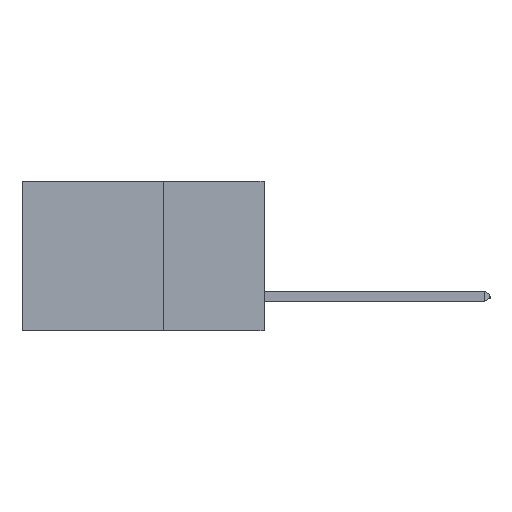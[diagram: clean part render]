
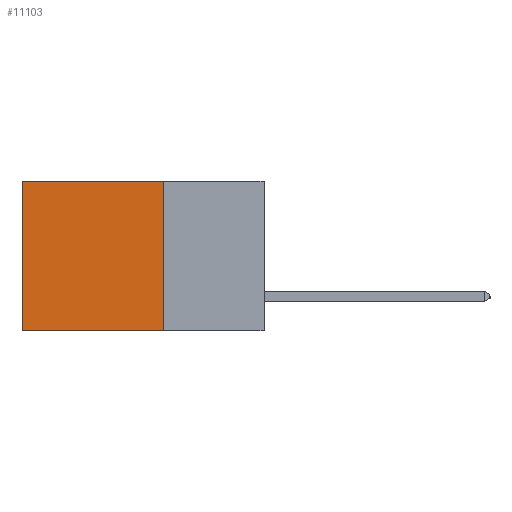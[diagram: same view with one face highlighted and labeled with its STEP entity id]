
A CAD part, left-side view. The second image highlights one B-rep face of the part: STEP entity #11103.
In plain terms, the highlighted planar face has unit normal (-1, 0, 0).
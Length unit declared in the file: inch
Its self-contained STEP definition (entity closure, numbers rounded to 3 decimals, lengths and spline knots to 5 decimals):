
#377 = DIRECTION ( 'NONE',  ( 1., 0., 0. ) ) ;
#1477 = VECTOR ( 'NONE', #22156, 39.37008 ) ;
#1693 = EDGE_CURVE ( 'NONE', #18777, #16874, #9585, .T. ) ;
#2269 = AXIS2_PLACEMENT_3D ( 'NONE', #9538, #377, #13287 ) ;
#2341 = CARTESIAN_POINT ( 'NONE',  ( 0.298, 0.25, 0. ) ) ;
#2598 = VERTEX_POINT ( 'NONE', #2831 ) ;
#2831 = CARTESIAN_POINT ( 'NONE',  ( 0.298, 0.25, -0.37 ) ) ;
#3844 = DIRECTION ( 'NONE',  ( 0., 1., 0. ) ) ;
#3929 = LINE ( 'NONE', #10751, #13177 ) ;
#4366 = CARTESIAN_POINT ( 'NONE',  ( 0.298, 0.25, 0. ) ) ;
#5441 = ORIENTED_EDGE ( 'NONE', *, *, #1693, .T. ) ;
#7174 = CARTESIAN_POINT ( 'NONE',  ( 0.298, 0.25, 0. ) ) ;
#7949 = EDGE_CURVE ( 'NONE', #16874, #20364, #11860, .T. ) ;
#8412 = EDGE_LOOP ( 'NONE', ( #9352, #10236, #23062, #5441 ) ) ;
#8668 = EDGE_CURVE ( 'NONE', #18777, #2598, #16421, .T. ) ;
#9352 = ORIENTED_EDGE ( 'NONE', *, *, #7949, .T. ) ;
#9538 = CARTESIAN_POINT ( 'NONE',  ( 0.298, 0.25, 0. ) ) ;
#9585 = LINE ( 'NONE', #7174, #19977 ) ;
#9738 = DIRECTION ( 'NONE',  ( 0., 0., -1. ) ) ;
#10236 = ORIENTED_EDGE ( 'NONE', *, *, #11571, .F. ) ;
#10751 = CARTESIAN_POINT ( 'NONE',  ( 0.298, 0.25, -0.37 ) ) ;
#10834 = FACE_OUTER_BOUND ( 'NONE', #8412, .T. ) ;
#11003 = CARTESIAN_POINT ( 'NONE',  ( 0.298, 0.6, -0.37 ) ) ;
#11103 = ADVANCED_FACE ( 'NONE', ( #10834 ), #11356, .F. ) ;
#11356 = PLANE ( 'NONE',  #2269 ) ;
#11516 = VECTOR ( 'NONE', #9738, 39.37008 ) ;
#11571 = EDGE_CURVE ( 'NONE', #2598, #20364, #3929, .T. ) ;
#11860 = LINE ( 'NONE', #20305, #1477 ) ;
#13177 = VECTOR ( 'NONE', #16250, 39.37008 ) ;
#13287 = DIRECTION ( 'NONE',  ( 0., 0., -1. ) ) ;
#13807 = CARTESIAN_POINT ( 'NONE',  ( 0.298, 0.6, 0. ) ) ;
#16250 = DIRECTION ( 'NONE',  ( 0., 1., 0. ) ) ;
#16421 = LINE ( 'NONE', #2341, #11516 ) ;
#16874 = VERTEX_POINT ( 'NONE', #13807 ) ;
#18777 = VERTEX_POINT ( 'NONE', #4366 ) ;
#19977 = VECTOR ( 'NONE', #3844, 39.37008 ) ;
#20305 = CARTESIAN_POINT ( 'NONE',  ( 0.298, 0.6, 0. ) ) ;
#20364 = VERTEX_POINT ( 'NONE', #11003 ) ;
#22156 = DIRECTION ( 'NONE',  ( 0., 0., -1. ) ) ;
#23062 = ORIENTED_EDGE ( 'NONE', *, *, #8668, .F. ) ;
